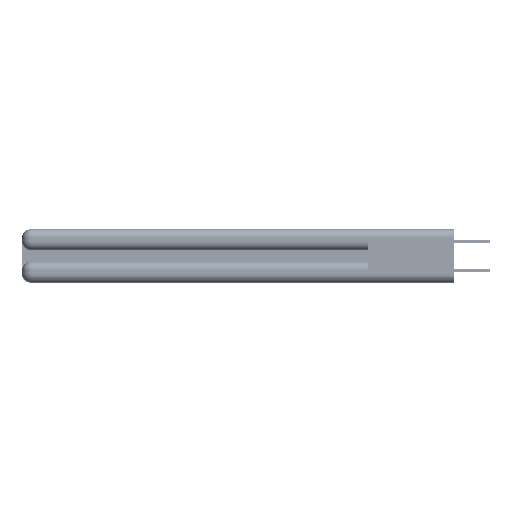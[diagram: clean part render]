
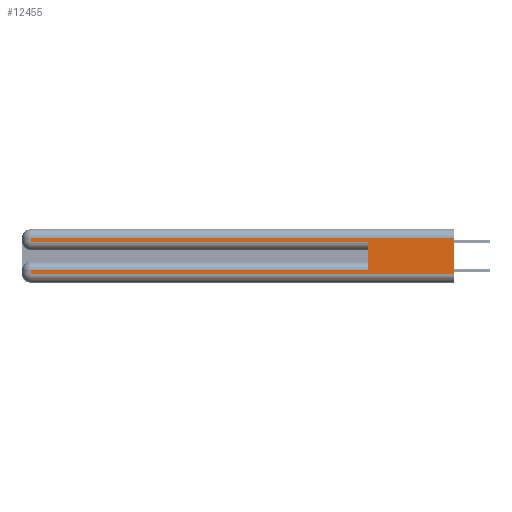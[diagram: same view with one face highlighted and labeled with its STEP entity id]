
A CAD part, left-side view. The second image highlights one B-rep face of the part: STEP entity #12455.
In plain terms, the highlighted planar face has unit normal (-1, 0, 0).
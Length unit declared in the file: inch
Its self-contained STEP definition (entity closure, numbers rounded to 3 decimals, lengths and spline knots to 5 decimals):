
#410 = LINE ( 'NONE', #26388, #19575 ) ;
#500 = ORIENTED_EDGE ( 'NONE', *, *, #19420, .T. ) ;
#1900 = VERTEX_POINT ( 'NONE', #31539 ) ;
#2270 = CARTESIAN_POINT ( 'NONE',  ( 0., 2.94, 0.285 ) ) ;
#3710 = VECTOR ( 'NONE', #4472, 39.37008 ) ;
#4472 = DIRECTION ( 'NONE',  ( 0., 1., 0. ) ) ;
#5319 = EDGE_CURVE ( 'NONE', #12574, #33454, #40282, .T. ) ;
#5793 = DIRECTION ( 'NONE',  ( 0., 0., -1. ) ) ;
#5941 = CARTESIAN_POINT ( 'NONE',  ( 0., 0., 0.085 ) ) ;
#6899 = VERTEX_POINT ( 'NONE', #15798 ) ;
#8294 = CARTESIAN_POINT ( 'NONE',  ( 0., 0., 0.06 ) ) ;
#8300 = DIRECTION ( 'NONE',  ( 0., 0., -1. ) ) ;
#8707 = DIRECTION ( 'NONE',  ( 0., 0., -1. ) ) ;
#9347 = EDGE_CURVE ( 'NONE', #16117, #42641, #25947, .T. ) ;
#10870 = EDGE_CURVE ( 'NONE', #29981, #33454, #32999, .T. ) ;
#11700 = CARTESIAN_POINT ( 'NONE',  ( 0., 0., 0.31 ) ) ;
#12434 = DIRECTION ( 'NONE',  ( 0., 1., 0. ) ) ;
#12455 = ADVANCED_FACE ( 'NONE', ( #22385 ), #32226, .F. ) ;
#12574 = VERTEX_POINT ( 'NONE', #2270 ) ;
#12612 = VECTOR ( 'NONE', #8300, 39.37008 ) ;
#12682 = EDGE_CURVE ( 'NONE', #1900, #30507, #19071, .T. ) ;
#12693 = VECTOR ( 'NONE', #19167, 39.37008 ) ;
#13246 = EDGE_CURVE ( 'NONE', #30507, #42641, #410, .T. ) ;
#14290 = CARTESIAN_POINT ( 'NONE',  ( 0., 0.6, 0.085 ) ) ;
#14457 = CARTESIAN_POINT ( 'NONE',  ( 0., 0., 0.285 ) ) ;
#14482 = VECTOR ( 'NONE', #38951, 39.37008 ) ;
#14736 = CARTESIAN_POINT ( 'NONE',  ( 0., 0., 0.37 ) ) ;
#15309 = LINE ( 'NONE', #39471, #12612 ) ;
#15798 = CARTESIAN_POINT ( 'NONE',  ( 0., 2.94, 0.31 ) ) ;
#15881 = ORIENTED_EDGE ( 'NONE', *, *, #13246, .T. ) ;
#16117 = VERTEX_POINT ( 'NONE', #16877 ) ;
#16877 = CARTESIAN_POINT ( 'NONE',  ( 0., 0., 0.31 ) ) ;
#16897 = ORIENTED_EDGE ( 'NONE', *, *, #10870, .F. ) ;
#16905 = ORIENTED_EDGE ( 'NONE', *, *, #9347, .F. ) ;
#18287 = DIRECTION ( 'NONE',  ( 1., 0., 0. ) ) ;
#19071 = LINE ( 'NONE', #31818, #40450 ) ;
#19167 = DIRECTION ( 'NONE',  ( 0., 0., 1. ) ) ;
#19420 = EDGE_CURVE ( 'NONE', #6899, #12574, #15309, .T. ) ;
#19575 = VECTOR ( 'NONE', #43756, 39.37008 ) ;
#19641 = ORIENTED_EDGE ( 'NONE', *, *, #30814, .T. ) ;
#20951 = EDGE_CURVE ( 'NONE', #16117, #6899, #27225, .T. ) ;
#22241 = VECTOR ( 'NONE', #12434, 39.37008 ) ;
#22385 = FACE_OUTER_BOUND ( 'NONE', #40093, .T. ) ;
#22722 = CARTESIAN_POINT ( 'NONE',  ( 0., 0.6, 0.145 ) ) ;
#23621 = ORIENTED_EDGE ( 'NONE', *, *, #5319, .T. ) ;
#24589 = CARTESIAN_POINT ( 'NONE',  ( 0., 2.94, 0.06 ) ) ;
#24959 = LINE ( 'NONE', #5941, #22241 ) ;
#25947 = LINE ( 'NONE', #31623, #33641 ) ;
#26388 = CARTESIAN_POINT ( 'NONE',  ( 0., 0., 0.06 ) ) ;
#27225 = LINE ( 'NONE', #11700, #3710 ) ;
#29981 = VERTEX_POINT ( 'NONE', #14290 ) ;
#30507 = VERTEX_POINT ( 'NONE', #24589 ) ;
#30814 = EDGE_CURVE ( 'NONE', #29981, #1900, #24959, .T. ) ;
#31539 = CARTESIAN_POINT ( 'NONE',  ( 0., 2.94, 0.085 ) ) ;
#31623 = CARTESIAN_POINT ( 'NONE',  ( 0., 0., 0.37 ) ) ;
#31818 = CARTESIAN_POINT ( 'NONE',  ( 0., 2.94, 0.37 ) ) ;
#32226 = PLANE ( 'NONE',  #32498 ) ;
#32498 = AXIS2_PLACEMENT_3D ( 'NONE', #14736, #18287, #39381 ) ;
#32999 = LINE ( 'NONE', #22722, #12693 ) ;
#33454 = VERTEX_POINT ( 'NONE', #36221 ) ;
#33641 = VECTOR ( 'NONE', #5793, 39.37008 ) ;
#36221 = CARTESIAN_POINT ( 'NONE',  ( 0., 0.6, 0.285 ) ) ;
#36795 = ORIENTED_EDGE ( 'NONE', *, *, #12682, .T. ) ;
#37778 = ORIENTED_EDGE ( 'NONE', *, *, #20951, .T. ) ;
#38951 = DIRECTION ( 'NONE',  ( 0., -1., 0. ) ) ;
#39381 = DIRECTION ( 'NONE',  ( 0., 0., -1. ) ) ;
#39471 = CARTESIAN_POINT ( 'NONE',  ( 0., 2.94, 0.37 ) ) ;
#40093 = EDGE_LOOP ( 'NONE', ( #16905, #37778, #500, #23621, #16897, #19641, #36795, #15881 ) ) ;
#40282 = LINE ( 'NONE', #14457, #14482 ) ;
#40450 = VECTOR ( 'NONE', #8707, 39.37008 ) ;
#42641 = VERTEX_POINT ( 'NONE', #8294 ) ;
#43756 = DIRECTION ( 'NONE',  ( 0., -1., 0. ) ) ;
